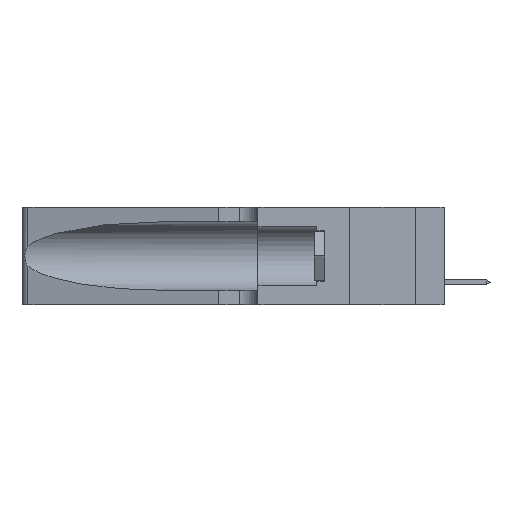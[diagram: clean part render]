
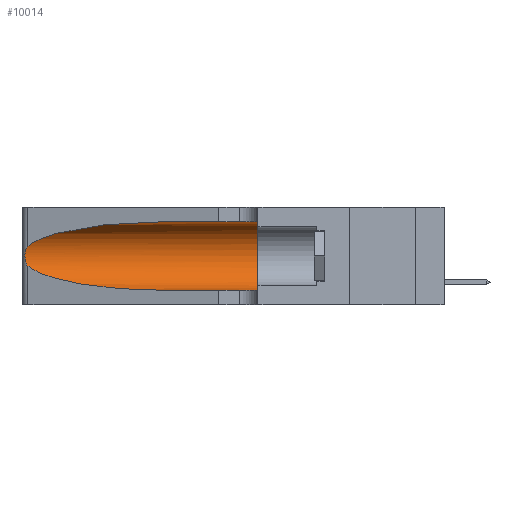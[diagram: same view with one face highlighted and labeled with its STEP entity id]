
A CAD part, left-side view. The second image highlights one B-rep face of the part: STEP entity #10014.
In plain terms, the highlighted cylindrical face has radius 3.308 mm (diameter 6.617 mm), a partial arc.
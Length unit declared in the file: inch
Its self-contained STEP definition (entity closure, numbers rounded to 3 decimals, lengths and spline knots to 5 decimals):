
#362 = CARTESIAN_POINT ( 'NONE',  ( 0.25487, 1.22718, 0.22369 ) ) ;
#831 = CARTESIAN_POINT ( 'NONE',  ( 0.25639, 1.23184, 0.21858 ) ) ;
#1127 = CARTESIAN_POINT ( 'NONE',  ( 0.1305, 0.72297, 0.05475 ) ) ;
#1128 = EDGE_CURVE ( 'NONE', #32669, #24776, #19032, .T. ) ;
#1143 = EDGE_CURVE ( 'NONE', #3388, #10328, #46027, .T. ) ;
#3276 = CARTESIAN_POINT ( 'NONE',  ( 0.25487, 1.22718, 0.22369 ) ) ;
#3388 = VERTEX_POINT ( 'NONE', #20159 ) ;
#4815 = AXIS2_PLACEMENT_3D ( 'NONE', #17379, #13158, #44421 ) ;
#5876 = EDGE_CURVE ( 'NONE', #10328, #32669, #45104, .T. ) ;
#8057 = CARTESIAN_POINT ( 'NONE',  ( 0.1305, 1.61858, 0.185 ) ) ;
#8316 = CARTESIAN_POINT ( 'NONE',  ( 0.25856, 1.23593, 0.16098 ) ) ;
#10014 = ADVANCED_FACE ( 'NONE', ( #42215 ), #11362, .F. ) ;
#10240 = VERTEX_POINT ( 'NONE', #24837 ) ;
#10328 = VERTEX_POINT ( 'NONE', #3276 ) ;
#11362 = CYLINDRICAL_SURFACE ( 'NONE', #26607, 0.13025 ) ;
#11899 = CARTESIAN_POINT ( 'NONE',  ( 0.25487, 1.22718, 0.14631 ) ) ;
#12249 = CARTESIAN_POINT ( 'NONE',  ( 0.25487, 1.22718, 0.14631 ) ) ;
#12576 = CARTESIAN_POINT ( 'NONE',  ( 0.26018, 1.23835, 0.19895 ) ) ;
#13158 = DIRECTION ( 'NONE',  ( 0., 1., 0. ) ) ;
#13717 = VERTEX_POINT ( 'NONE', #28275 ) ;
#14817 = CARTESIAN_POINT ( 'NONE',  ( 0.18966, 0.96281, 0.31525 ) ) ;
#15213 = CARTESIAN_POINT ( 'NONE',  ( 0.1305, 1.61858, 0.05475 ) ) ;
#15366 = DIRECTION ( 'NONE',  ( 0., -1., 0. ) ) ;
#15446 = ORIENTED_EDGE ( 'NONE', *, *, #32874, .F. ) ;
#16258 = CARTESIAN_POINT ( 'NONE',  ( 0.25787, 1.23484, 0.2124 ) ) ;
#16367 = CARTESIAN_POINT ( 'NONE',  ( 0.1305, 1.61858, 0.31525 ) ) ;
#17379 = CARTESIAN_POINT ( 'NONE',  ( 0.1305, 0.35, 0.185 ) ) ;
#19032 =( BOUNDED_CURVE ( )  B_SPLINE_CURVE ( 3, ( #11899, #39448, #43326, #48251 ),
 .UNSPECIFIED., .F., .F. ) 
 B_SPLINE_CURVE_WITH_KNOTS ( ( 4, 4 ),
 ( 3.44316, 4.71239 ),
 .UNSPECIFIED. ) 
 CURVE ( )  GEOMETRIC_REPRESENTATION_ITEM ( )  RATIONAL_B_SPLINE_CURVE ( ( 1., 0.87, 0.87, 1. ) ) 
 REPRESENTATION_ITEM ( '' )  );
#19687 = CARTESIAN_POINT ( 'NONE',  ( 0.25555, 1.22993, 0.14849 ) ) ;
#20159 = CARTESIAN_POINT ( 'NONE',  ( 0.1305, 0.72297, 0.31525 ) ) ;
#20167 = CARTESIAN_POINT ( 'NONE',  ( 0.25789, 1.23486, 0.15765 ) ) ;
#21335 = ORIENTED_EDGE ( 'NONE', *, *, #41344, .F. ) ;
#21801 = CARTESIAN_POINT ( 'NONE',  ( 0.25487, 1.22718, 0.14631 ) ) ;
#22162 = ORIENTED_EDGE ( 'NONE', *, *, #1128, .T. ) ;
#22947 = CARTESIAN_POINT ( 'NONE',  ( 0.1305, 0.72297, 0.31525 ) ) ;
#24168 = DIRECTION ( 'NONE',  ( 0., -1., 0. ) ) ;
#24776 = VERTEX_POINT ( 'NONE', #1127 ) ;
#24837 = CARTESIAN_POINT ( 'NONE',  ( 0.1305, 0.35, 0.05475 ) ) ;
#25447 = CARTESIAN_POINT ( 'NONE',  ( 0.25487, 1.22718, 0.22369 ) ) ;
#26607 = AXIS2_PLACEMENT_3D ( 'NONE', #8057, #39044, #46919 ) ;
#27165 = ORIENTED_EDGE ( 'NONE', *, *, #5876, .T. ) ;
#27285 = CIRCLE ( 'NONE', #4815, 0.13025 ) ;
#28275 = CARTESIAN_POINT ( 'NONE',  ( 0.1305, 0.35, 0.31525 ) ) ;
#29063 = VECTOR ( 'NONE', #24168, 39.37008 ) ;
#31809 = CARTESIAN_POINT ( 'NONE',  ( 0.25854, 1.2359, 0.20912 ) ) ;
#32669 = VERTEX_POINT ( 'NONE', #21801 ) ;
#32874 = EDGE_CURVE ( 'NONE', #13717, #10240, #27285, .T. ) ;
#34571 = CARTESIAN_POINT ( 'NONE',  ( 0.2373, 1.15595, 0.28018 ) ) ;
#35232 = CARTESIAN_POINT ( 'NONE',  ( 0.26075, 1.23896, 0.178 ) ) ;
#35392 = CARTESIAN_POINT ( 'NONE',  ( 0.25639, 1.23186, 0.15144 ) ) ;
#36608 = EDGE_LOOP ( 'NONE', ( #38795, #27165, #22162, #46442, #15446, #21335 ) ) ;
#36947 = LINE ( 'NONE', #16367, #29063 ) ;
#38795 = ORIENTED_EDGE ( 'NONE', *, *, #1143, .T. ) ;
#39044 = DIRECTION ( 'NONE',  ( 0., -1., 0. ) ) ;
#39448 = CARTESIAN_POINT ( 'NONE',  ( 0.2373, 1.15595, 0.08982 ) ) ;
#41159 = LINE ( 'NONE', #15213, #47047 ) ;
#41344 = EDGE_CURVE ( 'NONE', #3388, #13717, #36947, .T. ) ;
#42215 = FACE_OUTER_BOUND ( 'NONE', #36608, .T. ) ;
#42860 = CARTESIAN_POINT ( 'NONE',  ( 0.26075, 1.23896, 0.19203 ) ) ;
#43020 = CARTESIAN_POINT ( 'NONE',  ( 0.25555, 1.22994, 0.2215 ) ) ;
#43326 = CARTESIAN_POINT ( 'NONE',  ( 0.18966, 0.96281, 0.05475 ) ) ;
#43363 = CARTESIAN_POINT ( 'NONE',  ( 0.26017, 1.23833, 0.17102 ) ) ;
#44098 = EDGE_CURVE ( 'NONE', #24776, #10240, #41159, .T. ) ;
#44421 = DIRECTION ( 'NONE',  ( 0., 0., 1. ) ) ;
#45104 = B_SPLINE_CURVE_WITH_KNOTS ( 'NONE', 3,
 ( #362, #43020, #831, #16258, #31809, #12576, #42860, #35232, #43363, #8316, #20167, #35392, #19687, #12249 ),
 .UNSPECIFIED., .F., .F.,
 ( 4, 2, 2, 2, 2, 2, 4 ),
 ( 0., 0.00027, 0.00053, 0.00107, 0.0016, 0.00187, 0.00214 ),
 .UNSPECIFIED. ) ;
#46027 =( BOUNDED_CURVE ( )  B_SPLINE_CURVE ( 3, ( #22947, #14817, #34571, #25447 ),
 .UNSPECIFIED., .F., .F. ) 
 B_SPLINE_CURVE_WITH_KNOTS ( ( 4, 4 ),
 ( 1.5708, 2.84003 ),
 .UNSPECIFIED. ) 
 CURVE ( )  GEOMETRIC_REPRESENTATION_ITEM ( )  RATIONAL_B_SPLINE_CURVE ( ( 1., 0.87, 0.87, 1. ) ) 
 REPRESENTATION_ITEM ( '' )  );
#46442 = ORIENTED_EDGE ( 'NONE', *, *, #44098, .T. ) ;
#46919 = DIRECTION ( 'NONE',  ( 0., 0., -1. ) ) ;
#47047 = VECTOR ( 'NONE', #15366, 39.37008 ) ;
#48251 = CARTESIAN_POINT ( 'NONE',  ( 0.1305, 0.72297, 0.05475 ) ) ;
